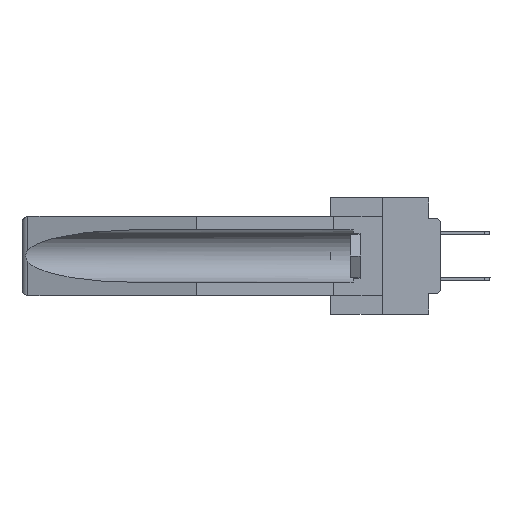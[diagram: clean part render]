
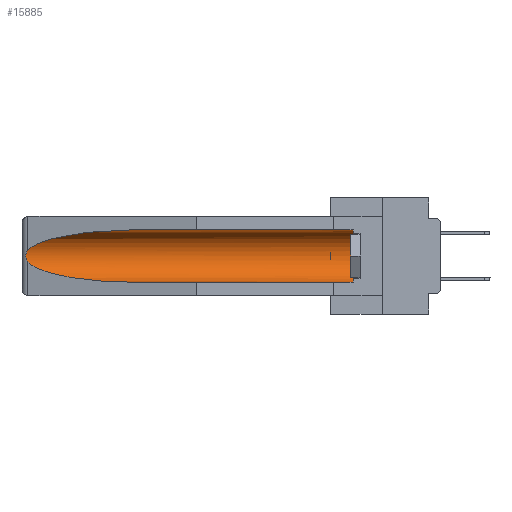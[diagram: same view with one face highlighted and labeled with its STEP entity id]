
A CAD part, left-side view. The second image highlights one B-rep face of the part: STEP entity #15885.
In plain terms, the highlighted cylindrical face has radius 2.857 mm (diameter 5.715 mm), a partial arc.
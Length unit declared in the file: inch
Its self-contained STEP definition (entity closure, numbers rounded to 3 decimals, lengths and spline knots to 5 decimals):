
#1256 = CARTESIAN_POINT ( 'NONE',  ( 0.155, -0.30754, -0.1715 ) ) ;
#1338 = EDGE_CURVE ( 'NONE', #25147, #19053, #8823, .T. ) ;
#2523 = DIRECTION ( 'NONE',  ( 0., 1., 0. ) ) ;
#3869 = ORIENTED_EDGE ( 'NONE', *, *, #38080, .T. ) ;
#3974 =( BOUNDED_CURVE ( )  B_SPLINE_CURVE ( 3, ( #39836, #5148, #4862, #21018 ),
 .UNSPECIFIED., .F., .F. ) 
 B_SPLINE_CURVE_WITH_KNOTS ( ( 4, 4 ),
 ( 0.1948, 1.5708 ),
 .UNSPECIFIED. ) 
 CURVE ( )  GEOMETRIC_REPRESENTATION_ITEM ( )  RATIONAL_B_SPLINE_CURVE ( ( 1., 0.848, 0.848, 1. ) ) 
 REPRESENTATION_ITEM ( '' )  );
#4080 = CARTESIAN_POINT ( 'NONE',  ( 0.26537, 1.52718, -0.14972 ) ) ;
#4219 = CARTESIAN_POINT ( 'NONE',  ( 0.2675, 1.53308, -0.16763 ) ) ;
#4460 = ORIENTED_EDGE ( 'NONE', *, *, #28865, .T. ) ;
#4713 = DIRECTION ( 'NONE',  ( 0., -1., 0. ) ) ;
#4862 = CARTESIAN_POINT ( 'NONE',  ( 0.21114, 1.30732, -0.284 ) ) ;
#5148 = CARTESIAN_POINT ( 'NONE',  ( 0.25451, 1.48313, -0.24835 ) ) ;
#5363 = DIRECTION ( 'NONE',  ( 0., 0., 1. ) ) ;
#8775 = VECTOR ( 'NONE', #39744, 39.37008 ) ;
#8823 = LINE ( 'NONE', #14678, #8775 ) ;
#9945 = CARTESIAN_POINT ( 'NONE',  ( 0.155, 0.126, -0.284 ) ) ;
#10796 = CARTESIAN_POINT ( 'NONE',  ( 0.26655, 1.53094, -0.18657 ) ) ;
#10927 = DIRECTION ( 'NONE',  ( 0., 1., 0. ) ) ;
#10948 = CARTESIAN_POINT ( 'NONE',  ( 0.26654, 1.53092, -0.15636 ) ) ;
#11817 = ORIENTED_EDGE ( 'NONE', *, *, #16659, .T. ) ;
#12122 = FACE_OUTER_BOUND ( 'NONE', #26316, .T. ) ;
#12830 = VERTEX_POINT ( 'NONE', #15283 ) ;
#13427 = CARTESIAN_POINT ( 'NONE',  ( 0.155, 1.07973, -0.059 ) ) ;
#14174 = AXIS2_PLACEMENT_3D ( 'NONE', #1256, #10927, #5363 ) ;
#14282 = VERTEX_POINT ( 'NONE', #25153 ) ;
#14678 = CARTESIAN_POINT ( 'NONE',  ( 0.155, -0.30754, -0.284 ) ) ;
#15283 = CARTESIAN_POINT ( 'NONE',  ( 0.26537, 1.52718, -0.19328 ) ) ;
#15607 = CYLINDRICAL_SURFACE ( 'NONE', #14174, 0.1125 ) ;
#15868 = VECTOR ( 'NONE', #2523, 39.37008 ) ;
#15885 = ADVANCED_FACE ( 'NONE', ( #12122 ), #15607, .F. ) ;
#16659 = EDGE_CURVE ( 'NONE', #28069, #26120, #26215, .T. ) ;
#19053 = VERTEX_POINT ( 'NONE', #32222 ) ;
#20234 = CARTESIAN_POINT ( 'NONE',  ( 0.26597, 1.5296, -0.19026 ) ) ;
#20599 = ORIENTED_EDGE ( 'NONE', *, *, #24378, .T. ) ;
#20881 = DIRECTION ( 'NONE',  ( 0., 0., 1. ) ) ;
#21018 = CARTESIAN_POINT ( 'NONE',  ( 0.155, 1.07973, -0.284 ) ) ;
#23059 = CARTESIAN_POINT ( 'NONE',  ( 0.2675, 1.53308, -0.17534 ) ) ;
#23215 = CARTESIAN_POINT ( 'NONE',  ( 0.26537, 1.52718, -0.14972 ) ) ;
#23324 = CARTESIAN_POINT ( 'NONE',  ( 0.26597, 1.52961, -0.15275 ) ) ;
#24378 = EDGE_CURVE ( 'NONE', #25147, #14282, #34134, .T. ) ;
#25147 = VERTEX_POINT ( 'NONE', #9945 ) ;
#25153 = CARTESIAN_POINT ( 'NONE',  ( 0.155, 0.126, -0.059 ) ) ;
#25320 = ORIENTED_EDGE ( 'NONE', *, *, #29839, .T. ) ;
#25369 = CARTESIAN_POINT ( 'NONE',  ( 0.26537, 1.52718, -0.14972 ) ) ;
#26120 = VERTEX_POINT ( 'NONE', #25369 ) ;
#26215 =( BOUNDED_CURVE ( )  B_SPLINE_CURVE ( 3, ( #13427, #29618, #30474, #23215 ),
 .UNSPECIFIED., .F., .F. ) 
 B_SPLINE_CURVE_WITH_KNOTS ( ( 4, 4 ),
 ( 4.71239, 6.08839 ),
 .UNSPECIFIED. ) 
 CURVE ( )  GEOMETRIC_REPRESENTATION_ITEM ( )  RATIONAL_B_SPLINE_CURVE ( ( 1., 0.848, 0.848, 1. ) ) 
 REPRESENTATION_ITEM ( '' )  );
#26316 = EDGE_LOOP ( 'NONE', ( #11817, #3869, #4460, #35932, #20599, #25320 ) ) ;
#28069 = VERTEX_POINT ( 'NONE', #36500 ) ;
#28865 = EDGE_CURVE ( 'NONE', #12830, #19053, #3974, .T. ) ;
#29378 = AXIS2_PLACEMENT_3D ( 'NONE', #39842, #4713, #20881 ) ;
#29589 = CARTESIAN_POINT ( 'NONE',  ( 0.2673, 1.5327, -0.16383 ) ) ;
#29618 = CARTESIAN_POINT ( 'NONE',  ( 0.21114, 1.30732, -0.059 ) ) ;
#29839 = EDGE_CURVE ( 'NONE', #14282, #28069, #40813, .T. ) ;
#29875 = CARTESIAN_POINT ( 'NONE',  ( 0.2673, 1.53269, -0.17917 ) ) ;
#30474 = CARTESIAN_POINT ( 'NONE',  ( 0.25451, 1.48313, -0.09465 ) ) ;
#32222 = CARTESIAN_POINT ( 'NONE',  ( 0.155, 1.07973, -0.284 ) ) ;
#34134 = CIRCLE ( 'NONE', #29378, 0.1125 ) ;
#35913 = CARTESIAN_POINT ( 'NONE',  ( 0.26537, 1.52718, -0.19328 ) ) ;
#35932 = ORIENTED_EDGE ( 'NONE', *, *, #1338, .F. ) ;
#36500 = CARTESIAN_POINT ( 'NONE',  ( 0.155, 1.07973, -0.059 ) ) ;
#37705 = B_SPLINE_CURVE_WITH_KNOTS ( 'NONE', 3,
 ( #4080, #23324, #10948, #29589, #4219, #23059, #29875, #10796, #20234, #35913 ),
 .UNSPECIFIED., .F., .F.,
 ( 4, 2, 2, 2, 4 ),
 ( 0., 0.00029, 0.00058, 0.00087, 0.00117 ),
 .UNSPECIFIED. ) ;
#38080 = EDGE_CURVE ( 'NONE', #26120, #12830, #37705, .T. ) ;
#39744 = DIRECTION ( 'NONE',  ( 0., 1., 0. ) ) ;
#39836 = CARTESIAN_POINT ( 'NONE',  ( 0.26537, 1.52718, -0.19328 ) ) ;
#39842 = CARTESIAN_POINT ( 'NONE',  ( 0.155, 0.126, -0.1715 ) ) ;
#40722 = CARTESIAN_POINT ( 'NONE',  ( 0.155, -0.30754, -0.059 ) ) ;
#40813 = LINE ( 'NONE', #40722, #15868 ) ;
